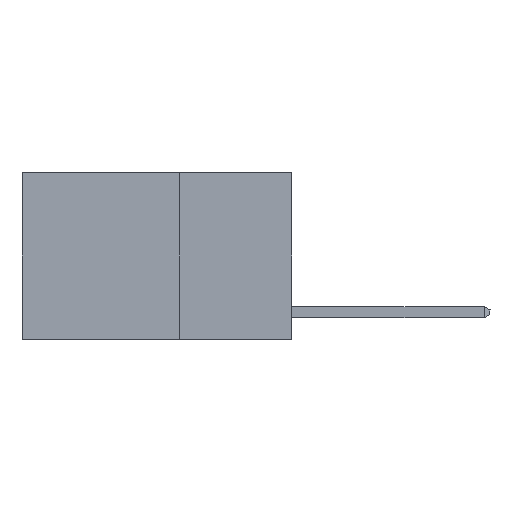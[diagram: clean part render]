
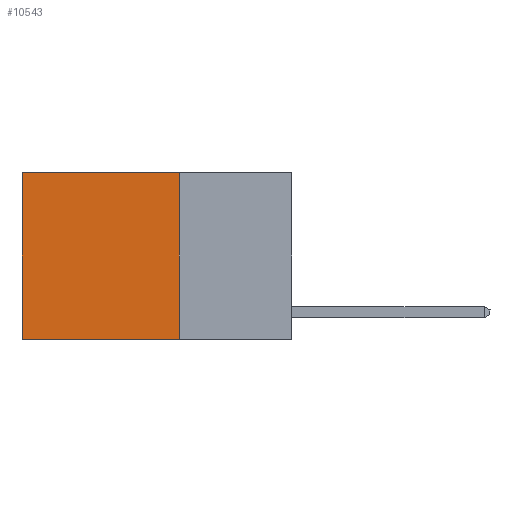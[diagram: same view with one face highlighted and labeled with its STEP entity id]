
A CAD part, left-side view. The second image highlights one B-rep face of the part: STEP entity #10543.
In plain terms, the highlighted planar face has unit normal (-1, 0, 0).
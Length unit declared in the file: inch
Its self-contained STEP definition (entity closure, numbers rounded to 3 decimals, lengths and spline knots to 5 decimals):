
#509 = DIRECTION ( 'NONE',  ( 1., 0., 0. ) ) ;
#2271 = LINE ( 'NONE', #10554, #5808 ) ;
#2367 = DIRECTION ( 'NONE',  ( 0., 0., -1. ) ) ;
#3001 = LINE ( 'NONE', #9866, #5802 ) ;
#3039 = CARTESIAN_POINT ( 'NONE',  ( 0.2625, 0.6, 0. ) ) ;
#4488 = CARTESIAN_POINT ( 'NONE',  ( 0.2625, 0.25, 0. ) ) ;
#4494 = EDGE_LOOP ( 'NONE', ( #5271, #8184, #5501, #9978 ) ) ;
#4547 = VECTOR ( 'NONE', #11999, 39.37008 ) ;
#5271 = ORIENTED_EDGE ( 'NONE', *, *, #9691, .T. ) ;
#5353 = FACE_OUTER_BOUND ( 'NONE', #4494, .T. ) ;
#5501 = ORIENTED_EDGE ( 'NONE', *, *, #6799, .F. ) ;
#5802 = VECTOR ( 'NONE', #7890, 39.37008 ) ;
#5808 = VECTOR ( 'NONE', #10366, 39.37008 ) ;
#6040 = CARTESIAN_POINT ( 'NONE',  ( 0.2625, 0.25, -0.37 ) ) ;
#6074 = PLANE ( 'NONE',  #8539 ) ;
#6799 = EDGE_CURVE ( 'NONE', #9721, #10587, #7335, .T. ) ;
#7025 = CARTESIAN_POINT ( 'NONE',  ( 0.2625, 0.25, -0.37 ) ) ;
#7335 = LINE ( 'NONE', #4488, #4547 ) ;
#7890 = DIRECTION ( 'NONE',  ( 0., 1., 0. ) ) ;
#8184 = ORIENTED_EDGE ( 'NONE', *, *, #8497, .F. ) ;
#8497 = EDGE_CURVE ( 'NONE', #10587, #9683, #8924, .T. ) ;
#8539 = AXIS2_PLACEMENT_3D ( 'NONE', #10923, #509, #2367 ) ;
#8924 = LINE ( 'NONE', #7025, #10989 ) ;
#9134 = CARTESIAN_POINT ( 'NONE',  ( 0.2625, 0.25, 0. ) ) ;
#9683 = VERTEX_POINT ( 'NONE', #11442 ) ;
#9691 = EDGE_CURVE ( 'NONE', #9697, #9683, #2271, .T. ) ;
#9697 = VERTEX_POINT ( 'NONE', #3039 ) ;
#9721 = VERTEX_POINT ( 'NONE', #9134 ) ;
#9866 = CARTESIAN_POINT ( 'NONE',  ( 0.2625, 0.25, 0. ) ) ;
#9978 = ORIENTED_EDGE ( 'NONE', *, *, #11040, .T. ) ;
#10366 = DIRECTION ( 'NONE',  ( 0., 0., -1. ) ) ;
#10543 = ADVANCED_FACE ( 'NONE', ( #5353 ), #6074, .F. ) ;
#10554 = CARTESIAN_POINT ( 'NONE',  ( 0.2625, 0.6, 0. ) ) ;
#10587 = VERTEX_POINT ( 'NONE', #6040 ) ;
#10923 = CARTESIAN_POINT ( 'NONE',  ( 0.2625, 0.25, 0. ) ) ;
#10989 = VECTOR ( 'NONE', #11755, 39.37008 ) ;
#11040 = EDGE_CURVE ( 'NONE', #9721, #9697, #3001, .T. ) ;
#11442 = CARTESIAN_POINT ( 'NONE',  ( 0.2625, 0.6, -0.37 ) ) ;
#11755 = DIRECTION ( 'NONE',  ( 0., 1., 0. ) ) ;
#11999 = DIRECTION ( 'NONE',  ( 0., 0., -1. ) ) ;
